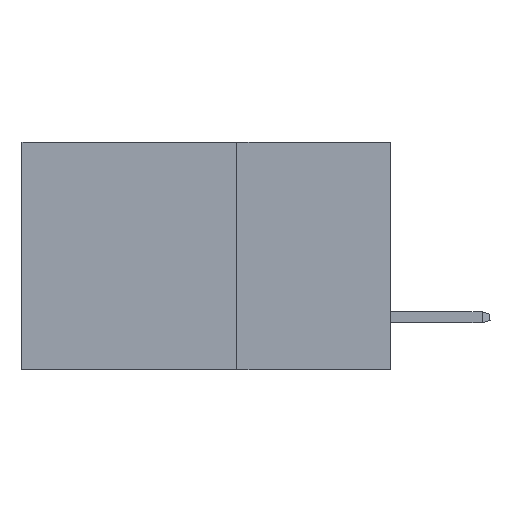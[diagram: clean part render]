
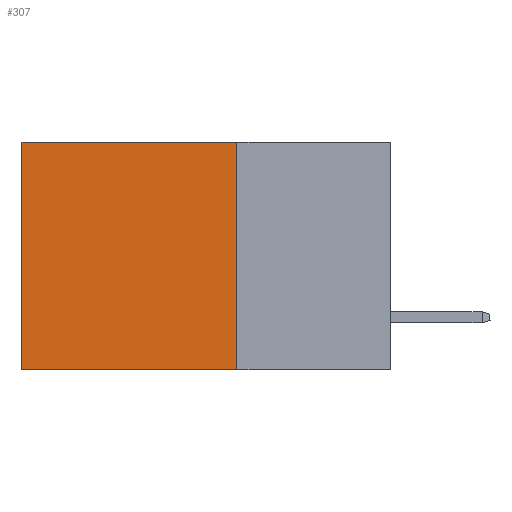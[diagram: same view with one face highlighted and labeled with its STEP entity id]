
A CAD part, left-side view. The second image highlights one B-rep face of the part: STEP entity #307.
In plain terms, the highlighted planar face has unit normal (-1, 0, 0).
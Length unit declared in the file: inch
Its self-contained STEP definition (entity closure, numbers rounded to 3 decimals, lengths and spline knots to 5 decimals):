
#307 = ADVANCED_FACE ( 'NONE', ( #12612 ), #14935, .F. ) ;
#1028 = VECTOR ( 'NONE', #13251, 39.37008 ) ;
#1132 = VECTOR ( 'NONE', #14580, 39.37008 ) ;
#1136 = VERTEX_POINT ( 'NONE', #11521 ) ;
#1580 = VECTOR ( 'NONE', #10262, 39.37008 ) ;
#1625 = ORIENTED_EDGE ( 'NONE', *, *, #15050, .F. ) ;
#2509 = DIRECTION ( 'NONE',  ( 0., 0., -1. ) ) ;
#2922 = VERTEX_POINT ( 'NONE', #13242 ) ;
#3679 = DIRECTION ( 'NONE',  ( 1., 0., 0. ) ) ;
#4031 = CARTESIAN_POINT ( 'NONE',  ( 0.2875, 0.25, -0.37 ) ) ;
#4487 = CARTESIAN_POINT ( 'NONE',  ( 0.2875, 0.25, -0.37 ) ) ;
#4749 = ORIENTED_EDGE ( 'NONE', *, *, #7293, .F. ) ;
#4971 = CARTESIAN_POINT ( 'NONE',  ( 0.2875, 0.25, 0. ) ) ;
#6174 = LINE ( 'NONE', #4487, #1028 ) ;
#6320 = VERTEX_POINT ( 'NONE', #10740 ) ;
#6836 = CARTESIAN_POINT ( 'NONE',  ( 0.2875, 0.6, 0. ) ) ;
#7293 = EDGE_CURVE ( 'NONE', #12565, #1136, #6174, .T. ) ;
#8122 = EDGE_CURVE ( 'NONE', #6320, #1136, #9464, .T. ) ;
#8210 = CARTESIAN_POINT ( 'NONE',  ( 0.2875, 0.25, 0. ) ) ;
#8553 = ORIENTED_EDGE ( 'NONE', *, *, #8122, .T. ) ;
#9464 = LINE ( 'NONE', #6836, #1580 ) ;
#10262 = DIRECTION ( 'NONE',  ( 0., 0., -1. ) ) ;
#10740 = CARTESIAN_POINT ( 'NONE',  ( 0.2875, 0.6, 0. ) ) ;
#11521 = CARTESIAN_POINT ( 'NONE',  ( 0.2875, 0.6, -0.37 ) ) ;
#11726 = AXIS2_PLACEMENT_3D ( 'NONE', #13654, #3679, #2509 ) ;
#11973 = VECTOR ( 'NONE', #12481, 39.37008 ) ;
#12372 = LINE ( 'NONE', #4971, #11973 ) ;
#12481 = DIRECTION ( 'NONE',  ( 0., 1., 0. ) ) ;
#12565 = VERTEX_POINT ( 'NONE', #4031 ) ;
#12612 = FACE_OUTER_BOUND ( 'NONE', #13754, .T. ) ;
#13242 = CARTESIAN_POINT ( 'NONE',  ( 0.2875, 0.25, 0. ) ) ;
#13251 = DIRECTION ( 'NONE',  ( 0., 1., 0. ) ) ;
#13654 = CARTESIAN_POINT ( 'NONE',  ( 0.2875, 0.25, 0. ) ) ;
#13754 = EDGE_LOOP ( 'NONE', ( #8553, #4749, #1625, #16026 ) ) ;
#14298 = EDGE_CURVE ( 'NONE', #2922, #6320, #12372, .T. ) ;
#14580 = DIRECTION ( 'NONE',  ( 0., 0., -1. ) ) ;
#14935 = PLANE ( 'NONE',  #11726 ) ;
#15050 = EDGE_CURVE ( 'NONE', #2922, #12565, #15277, .T. ) ;
#15277 = LINE ( 'NONE', #8210, #1132 ) ;
#16026 = ORIENTED_EDGE ( 'NONE', *, *, #14298, .T. ) ;
